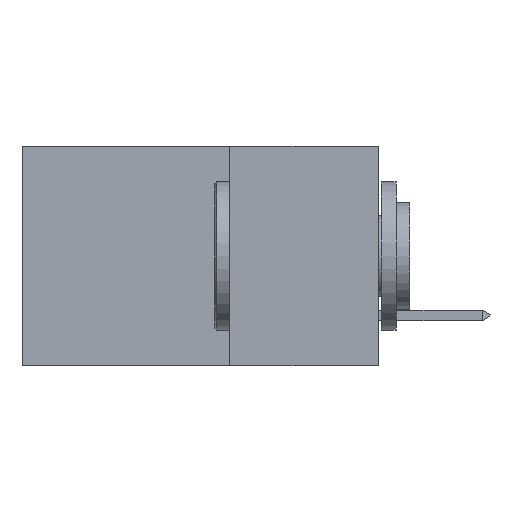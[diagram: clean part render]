
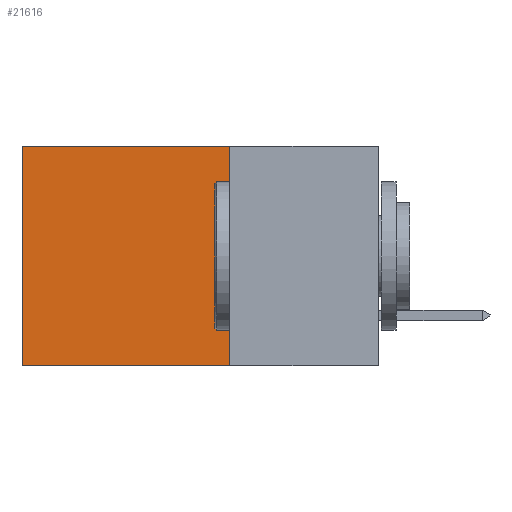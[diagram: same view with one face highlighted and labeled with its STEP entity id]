
A CAD part, left-side view. The second image highlights one B-rep face of the part: STEP entity #21616.
In plain terms, the highlighted planar face has unit normal (-1, 0, 0).
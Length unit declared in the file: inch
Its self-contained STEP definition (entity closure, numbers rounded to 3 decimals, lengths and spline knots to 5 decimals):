
#25 = LINE ( 'NONE', #19292, #1079 ) ;
#36 = VERTEX_POINT ( 'NONE', #5303 ) ;
#1079 = VECTOR ( 'NONE', #16129, 39.37008 ) ;
#1773 = CARTESIAN_POINT ( 'NONE',  ( 0.2615, 0.25, -0.37 ) ) ;
#2265 = EDGE_LOOP ( 'NONE', ( #10121, #11008, #16759, #18848 ) ) ;
#3257 = EDGE_CURVE ( 'NONE', #22022, #22109, #20705, .T. ) ;
#4581 = AXIS2_PLACEMENT_3D ( 'NONE', #11070, #17076, #9981 ) ;
#5303 = CARTESIAN_POINT ( 'NONE',  ( 0.2615, 0.6, 0. ) ) ;
#6166 = CARTESIAN_POINT ( 'NONE',  ( 0.2615, 0.25, 0. ) ) ;
#7577 = PLANE ( 'NONE',  #4581 ) ;
#9864 = EDGE_CURVE ( 'NONE', #22109, #16311, #21159, .T. ) ;
#9981 = DIRECTION ( 'NONE',  ( 0., 0., -1. ) ) ;
#10121 = ORIENTED_EDGE ( 'NONE', *, *, #15388, .T. ) ;
#10718 = LINE ( 'NONE', #6166, #11591 ) ;
#11008 = ORIENTED_EDGE ( 'NONE', *, *, #9864, .F. ) ;
#11070 = CARTESIAN_POINT ( 'NONE',  ( 0.2615, 0.25, -0.37 ) ) ;
#11591 = VECTOR ( 'NONE', #20496, 39.37008 ) ;
#12120 = CARTESIAN_POINT ( 'NONE',  ( 0.2615, 0.6, -0.37 ) ) ;
#13288 = CARTESIAN_POINT ( 'NONE',  ( 0.2615, 0.25, 0. ) ) ;
#13632 = VECTOR ( 'NONE', #21633, 39.37008 ) ;
#15388 = EDGE_CURVE ( 'NONE', #36, #16311, #25, .T. ) ;
#15448 = DIRECTION ( 'NONE',  ( 0., 0., -1. ) ) ;
#16129 = DIRECTION ( 'NONE',  ( 0., 0., -1. ) ) ;
#16311 = VERTEX_POINT ( 'NONE', #12120 ) ;
#16461 = VECTOR ( 'NONE', #15448, 39.37008 ) ;
#16759 = ORIENTED_EDGE ( 'NONE', *, *, #3257, .F. ) ;
#17076 = DIRECTION ( 'NONE',  ( 1., 0., 0. ) ) ;
#18848 = ORIENTED_EDGE ( 'NONE', *, *, #19960, .T. ) ;
#19064 = CARTESIAN_POINT ( 'NONE',  ( 0.2615, 0.25, -0.37 ) ) ;
#19292 = CARTESIAN_POINT ( 'NONE',  ( 0.2615, 0.6, -0.37 ) ) ;
#19938 = FACE_OUTER_BOUND ( 'NONE', #2265, .T. ) ;
#19960 = EDGE_CURVE ( 'NONE', #22022, #36, #10718, .T. ) ;
#20496 = DIRECTION ( 'NONE',  ( 0., 1., 0. ) ) ;
#20705 = LINE ( 'NONE', #19064, #16461 ) ;
#20882 = CARTESIAN_POINT ( 'NONE',  ( 0.2615, 0.25, -0.37 ) ) ;
#21159 = LINE ( 'NONE', #1773, #13632 ) ;
#21616 = ADVANCED_FACE ( 'NONE', ( #19938 ), #7577, .F. ) ;
#21633 = DIRECTION ( 'NONE',  ( 0., 1., 0. ) ) ;
#22022 = VERTEX_POINT ( 'NONE', #13288 ) ;
#22109 = VERTEX_POINT ( 'NONE', #20882 ) ;
